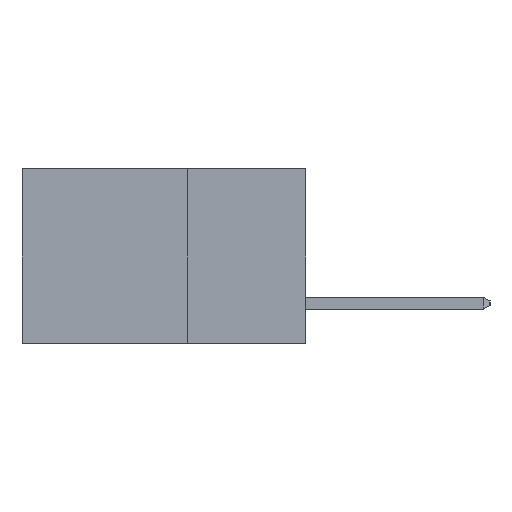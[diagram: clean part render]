
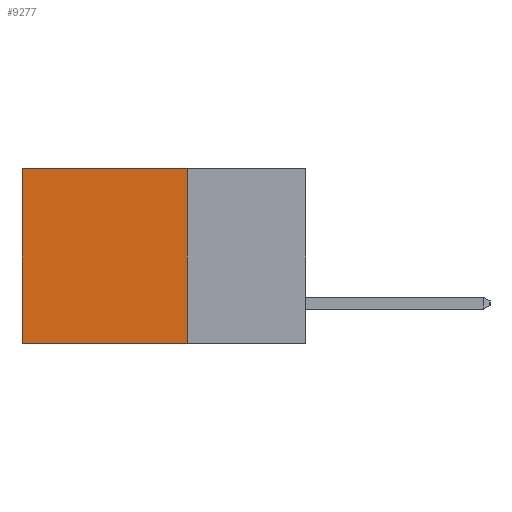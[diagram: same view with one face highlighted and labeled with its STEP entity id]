
A CAD part, left-side view. The second image highlights one B-rep face of the part: STEP entity #9277.
In plain terms, the highlighted planar face has unit normal (-1, 0, 0).
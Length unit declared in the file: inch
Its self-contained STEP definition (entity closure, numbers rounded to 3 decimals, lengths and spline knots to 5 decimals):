
#291 = EDGE_CURVE ( 'NONE', #5286, #6569, #3567, .T. ) ;
#783 = ORIENTED_EDGE ( 'NONE', *, *, #8031, .F. ) ;
#972 = CARTESIAN_POINT ( 'NONE',  ( 0.2615, 0.25, 0. ) ) ;
#1027 = FACE_OUTER_BOUND ( 'NONE', #6059, .T. ) ;
#1141 = EDGE_CURVE ( 'NONE', #6569, #6563, #4044, .T. ) ;
#1448 = VERTEX_POINT ( 'NONE', #5493 ) ;
#1457 = DIRECTION ( 'NONE',  ( 1., 0., 0. ) ) ;
#2029 = CARTESIAN_POINT ( 'NONE',  ( 0.2615, 0.25, 0. ) ) ;
#2196 = CARTESIAN_POINT ( 'NONE',  ( 0.2615, 0.25, -0.37 ) ) ;
#2218 = ORIENTED_EDGE ( 'NONE', *, *, #1141, .T. ) ;
#2291 = EDGE_CURVE ( 'NONE', #5286, #1448, #7845, .T. ) ;
#2805 = AXIS2_PLACEMENT_3D ( 'NONE', #2196, #1457, #7009 ) ;
#3088 = ORIENTED_EDGE ( 'NONE', *, *, #2291, .F. ) ;
#3567 = LINE ( 'NONE', #2029, #5441 ) ;
#3622 = DIRECTION ( 'NONE',  ( 0., 1., 0. ) ) ;
#3662 = VECTOR ( 'NONE', #9828, 39.37008 ) ;
#4044 = LINE ( 'NONE', #7437, #7990 ) ;
#4139 = CARTESIAN_POINT ( 'NONE',  ( 0.2615, 0.6, -0.37 ) ) ;
#5286 = VERTEX_POINT ( 'NONE', #972 ) ;
#5313 = CARTESIAN_POINT ( 'NONE',  ( 0.2615, 0.25, -0.37 ) ) ;
#5441 = VECTOR ( 'NONE', #3622, 39.37008 ) ;
#5493 = CARTESIAN_POINT ( 'NONE',  ( 0.2615, 0.25, -0.37 ) ) ;
#5524 = VECTOR ( 'NONE', #6481, 39.37008 ) ;
#6018 = ORIENTED_EDGE ( 'NONE', *, *, #291, .T. ) ;
#6059 = EDGE_LOOP ( 'NONE', ( #2218, #783, #3088, #6018 ) ) ;
#6481 = DIRECTION ( 'NONE',  ( 0., 0., -1. ) ) ;
#6563 = VERTEX_POINT ( 'NONE', #4139 ) ;
#6569 = VERTEX_POINT ( 'NONE', #7273 ) ;
#7009 = DIRECTION ( 'NONE',  ( 0., 0., -1. ) ) ;
#7255 = CARTESIAN_POINT ( 'NONE',  ( 0.2615, 0.25, -0.37 ) ) ;
#7273 = CARTESIAN_POINT ( 'NONE',  ( 0.2615, 0.6, 0. ) ) ;
#7437 = CARTESIAN_POINT ( 'NONE',  ( 0.2615, 0.6, -0.37 ) ) ;
#7618 = LINE ( 'NONE', #5313, #3662 ) ;
#7845 = LINE ( 'NONE', #7255, #5524 ) ;
#7990 = VECTOR ( 'NONE', #8608, 39.37008 ) ;
#8031 = EDGE_CURVE ( 'NONE', #1448, #6563, #7618, .T. ) ;
#8608 = DIRECTION ( 'NONE',  ( 0., 0., -1. ) ) ;
#9248 = PLANE ( 'NONE',  #2805 ) ;
#9277 = ADVANCED_FACE ( 'NONE', ( #1027 ), #9248, .F. ) ;
#9828 = DIRECTION ( 'NONE',  ( 0., 1., 0. ) ) ;
